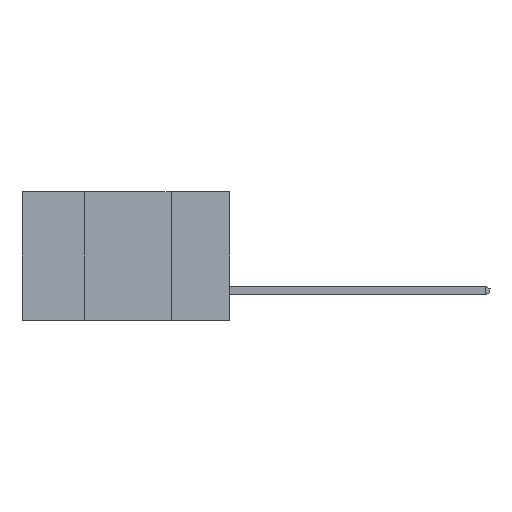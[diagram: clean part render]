
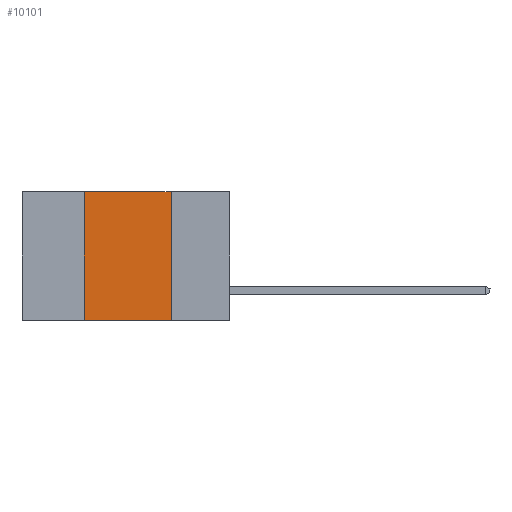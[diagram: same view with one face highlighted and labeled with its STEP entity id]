
A CAD part, left-side view. The second image highlights one B-rep face of the part: STEP entity #10101.
In plain terms, the highlighted planar face has unit normal (-1, 0, 0).
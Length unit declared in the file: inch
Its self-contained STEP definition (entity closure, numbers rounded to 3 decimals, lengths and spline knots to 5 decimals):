
#185 = LINE ( 'NONE', #249, #9841 ) ;
#249 = CARTESIAN_POINT ( 'NONE',  ( 0., 0.17, -0.37 ) ) ;
#288 = VERTEX_POINT ( 'NONE', #2352 ) ;
#1195 = DIRECTION ( 'NONE',  ( 0., -1., 0. ) ) ;
#2352 = CARTESIAN_POINT ( 'NONE',  ( 0., 0.42, 0. ) ) ;
#2737 = VERTEX_POINT ( 'NONE', #5631 ) ;
#3243 = VERTEX_POINT ( 'NONE', #8577 ) ;
#3966 = VECTOR ( 'NONE', #4676, 39.37008 ) ;
#4288 = EDGE_CURVE ( 'NONE', #3243, #2737, #10920, .T. ) ;
#4419 = AXIS2_PLACEMENT_3D ( 'NONE', #11150, #5457, #7418 ) ;
#4676 = DIRECTION ( 'NONE',  ( 0., 0., 1. ) ) ;
#5014 = CARTESIAN_POINT ( 'NONE',  ( 0., 0.17, 0. ) ) ;
#5457 = DIRECTION ( 'NONE',  ( 1., 0., 0. ) ) ;
#5631 = CARTESIAN_POINT ( 'NONE',  ( 0., 0.17, -0.37 ) ) ;
#7152 = EDGE_LOOP ( 'NONE', ( #7542, #9052, #10727, #9388 ) ) ;
#7400 = CARTESIAN_POINT ( 'NONE',  ( 0., 0.42, -0.37 ) ) ;
#7418 = DIRECTION ( 'NONE',  ( 0., 0., -1. ) ) ;
#7542 = ORIENTED_EDGE ( 'NONE', *, *, #8689, .F. ) ;
#7640 = EDGE_CURVE ( 'NONE', #288, #9591, #8284, .T. ) ;
#7939 = CARTESIAN_POINT ( 'NONE',  ( 0., 0.6, -0.37 ) ) ;
#8284 = LINE ( 'NONE', #9418, #11453 ) ;
#8361 = PLANE ( 'NONE',  #4419 ) ;
#8577 = CARTESIAN_POINT ( 'NONE',  ( 0., 0.42, -0.37 ) ) ;
#8689 = EDGE_CURVE ( 'NONE', #9591, #2737, #185, .T. ) ;
#8896 = EDGE_CURVE ( 'NONE', #3243, #288, #9420, .T. ) ;
#9052 = ORIENTED_EDGE ( 'NONE', *, *, #7640, .F. ) ;
#9354 = DIRECTION ( 'NONE',  ( 0., -1., 0. ) ) ;
#9388 = ORIENTED_EDGE ( 'NONE', *, *, #4288, .T. ) ;
#9418 = CARTESIAN_POINT ( 'NONE',  ( 0., 0.6, 0. ) ) ;
#9420 = LINE ( 'NONE', #7400, #3966 ) ;
#9591 = VERTEX_POINT ( 'NONE', #5014 ) ;
#9841 = VECTOR ( 'NONE', #11910, 39.37008 ) ;
#10101 = ADVANCED_FACE ( 'NONE', ( #10326 ), #8361, .F. ) ;
#10216 = VECTOR ( 'NONE', #1195, 39.37008 ) ;
#10326 = FACE_OUTER_BOUND ( 'NONE', #7152, .T. ) ;
#10727 = ORIENTED_EDGE ( 'NONE', *, *, #8896, .F. ) ;
#10920 = LINE ( 'NONE', #7939, #10216 ) ;
#11150 = CARTESIAN_POINT ( 'NONE',  ( 0., 0.6, 0. ) ) ;
#11453 = VECTOR ( 'NONE', #9354, 39.37008 ) ;
#11910 = DIRECTION ( 'NONE',  ( 0., 0., -1. ) ) ;
